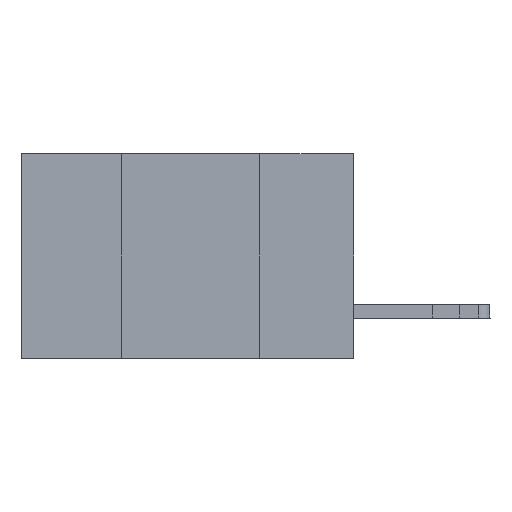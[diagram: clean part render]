
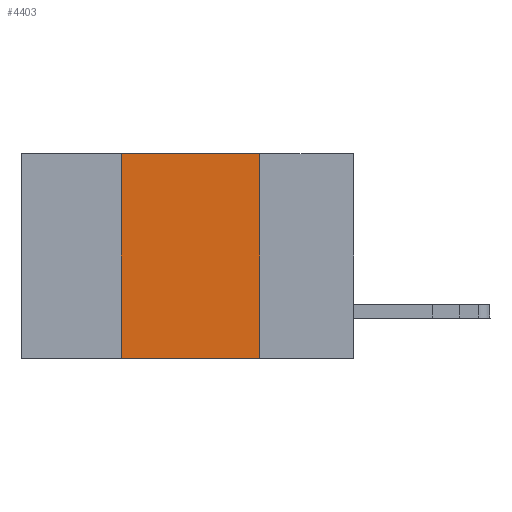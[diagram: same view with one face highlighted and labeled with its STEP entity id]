
A CAD part, left-side view. The second image highlights one B-rep face of the part: STEP entity #4403.
In plain terms, the highlighted planar face has unit normal (-1, 0, 0).
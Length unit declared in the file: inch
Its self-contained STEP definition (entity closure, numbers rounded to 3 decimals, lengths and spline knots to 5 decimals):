
#257 = EDGE_LOOP ( 'NONE', ( #19446, #3206, #10210, #11785 ) ) ;
#737 = CARTESIAN_POINT ( 'NONE',  ( 0., 0.17, 0. ) ) ;
#1475 = VERTEX_POINT ( 'NONE', #737 ) ;
#3206 = ORIENTED_EDGE ( 'NONE', *, *, #18198, .F. ) ;
#3709 = DIRECTION ( 'NONE',  ( 0., -1., 0. ) ) ;
#3764 = CARTESIAN_POINT ( 'NONE',  ( 0., 0.42, 0. ) ) ;
#4403 = ADVANCED_FACE ( 'NONE', ( #7560 ), #23019, .F. ) ;
#5561 = DIRECTION ( 'NONE',  ( 0., -1., 0. ) ) ;
#7306 = CARTESIAN_POINT ( 'NONE',  ( 0., 0.42, 0. ) ) ;
#7560 = FACE_OUTER_BOUND ( 'NONE', #257, .T. ) ;
#7636 = CARTESIAN_POINT ( 'NONE',  ( 0., 0.6, -0.37 ) ) ;
#7930 = VECTOR ( 'NONE', #18795, 39.37008 ) ;
#9332 = LINE ( 'NONE', #7306, #21186 ) ;
#9809 = DIRECTION ( 'NONE',  ( 0., 0., -1. ) ) ;
#10210 = ORIENTED_EDGE ( 'NONE', *, *, #23768, .F. ) ;
#10211 = VECTOR ( 'NONE', #3709, 39.37008 ) ;
#10420 = EDGE_CURVE ( 'NONE', #1475, #18342, #12548, .T. ) ;
#11491 = CARTESIAN_POINT ( 'NONE',  ( 0., 0.17, -0.37 ) ) ;
#11785 = ORIENTED_EDGE ( 'NONE', *, *, #18758, .T. ) ;
#12548 = LINE ( 'NONE', #16430, #7930 ) ;
#12667 = VERTEX_POINT ( 'NONE', #3764 ) ;
#13495 = CARTESIAN_POINT ( 'NONE',  ( 0., 0.6, 0. ) ) ;
#15237 = DIRECTION ( 'NONE',  ( 0., 0., 1. ) ) ;
#15629 = CARTESIAN_POINT ( 'NONE',  ( 0., 0.42, -0.37 ) ) ;
#16430 = CARTESIAN_POINT ( 'NONE',  ( 0., 0.17, 0. ) ) ;
#18198 = EDGE_CURVE ( 'NONE', #12667, #1475, #18767, .T. ) ;
#18342 = VERTEX_POINT ( 'NONE', #11491 ) ;
#18758 = EDGE_CURVE ( 'NONE', #19792, #18342, #20976, .T. ) ;
#18767 = LINE ( 'NONE', #18898, #21443 ) ;
#18795 = DIRECTION ( 'NONE',  ( 0., 0., -1. ) ) ;
#18898 = CARTESIAN_POINT ( 'NONE',  ( 0., 0.6, 0. ) ) ;
#19446 = ORIENTED_EDGE ( 'NONE', *, *, #10420, .F. ) ;
#19792 = VERTEX_POINT ( 'NONE', #15629 ) ;
#20976 = LINE ( 'NONE', #7636, #10211 ) ;
#21186 = VECTOR ( 'NONE', #15237, 39.37008 ) ;
#21443 = VECTOR ( 'NONE', #5561, 39.37008 ) ;
#22790 = DIRECTION ( 'NONE',  ( 1., 0., 0. ) ) ;
#23019 = PLANE ( 'NONE',  #23191 ) ;
#23191 = AXIS2_PLACEMENT_3D ( 'NONE', #13495, #22790, #9809 ) ;
#23768 = EDGE_CURVE ( 'NONE', #19792, #12667, #9332, .T. ) ;
